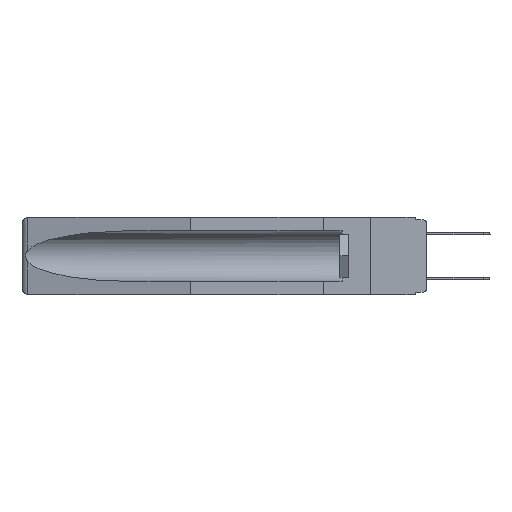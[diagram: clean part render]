
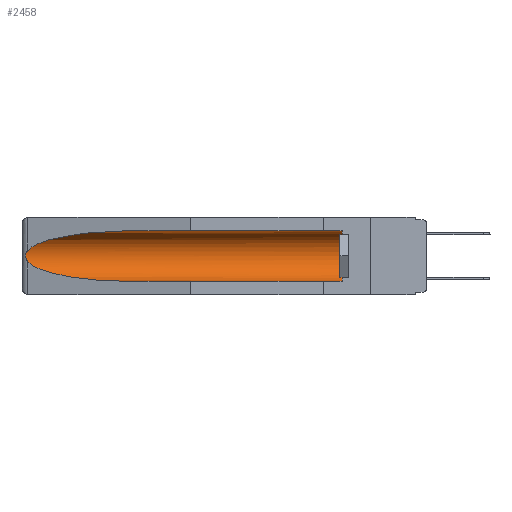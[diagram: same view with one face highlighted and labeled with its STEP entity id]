
A CAD part, left-side view. The second image highlights one B-rep face of the part: STEP entity #2458.
In plain terms, the highlighted cylindrical face has radius 2.857 mm (diameter 5.715 mm), a partial arc.
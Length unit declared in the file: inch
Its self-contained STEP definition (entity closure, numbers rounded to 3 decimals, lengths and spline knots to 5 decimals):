
#445 = CARTESIAN_POINT ( 'NONE',  ( 0.26537, 1.52718, -0.14972 ) ) ;
#566 = CARTESIAN_POINT ( 'NONE',  ( 0.26537, 1.52718, -0.19328 ) ) ;
#662 = VERTEX_POINT ( 'NONE', #4164 ) ;
#961 = EDGE_CURVE ( 'NONE', #3886, #20396, #15527, .T. ) ;
#1002 = CARTESIAN_POINT ( 'NONE',  ( 0.26654, 1.53092, -0.15636 ) ) ;
#1041 = ORIENTED_EDGE ( 'NONE', *, *, #12779, .T. ) ;
#1281 = CARTESIAN_POINT ( 'NONE',  ( 0.155, -0.30754, -0.059 ) ) ;
#2283 = FACE_OUTER_BOUND ( 'NONE', #13771, .T. ) ;
#2370 = ORIENTED_EDGE ( 'NONE', *, *, #7186, .T. ) ;
#2458 = ADVANCED_FACE ( 'NONE', ( #2283 ), #17508, .F. ) ;
#2615 = CARTESIAN_POINT ( 'NONE',  ( 0.155, 1.07973, -0.059 ) ) ;
#2893 = CARTESIAN_POINT ( 'NONE',  ( 0.26597, 1.52961, -0.15275 ) ) ;
#3886 = VERTEX_POINT ( 'NONE', #566 ) ;
#3907 = ORIENTED_EDGE ( 'NONE', *, *, #9377, .F. ) ;
#4164 = CARTESIAN_POINT ( 'NONE',  ( 0.155, 1.07973, -0.059 ) ) ;
#4908 = CARTESIAN_POINT ( 'NONE',  ( 0.26537, 1.52718, -0.14972 ) ) ;
#4993 = CARTESIAN_POINT ( 'NONE',  ( 0.2673, 1.5327, -0.16383 ) ) ;
#7072 = CARTESIAN_POINT ( 'NONE',  ( 0.26655, 1.53094, -0.18657 ) ) ;
#7186 = EDGE_CURVE ( 'NONE', #8641, #662, #25061, .T. ) ;
#7592 = CARTESIAN_POINT ( 'NONE',  ( 0.21114, 1.30732, -0.284 ) ) ;
#8641 = VERTEX_POINT ( 'NONE', #8971 ) ;
#8808 = LINE ( 'NONE', #23559, #21740 ) ;
#8971 = CARTESIAN_POINT ( 'NONE',  ( 0.155, 0.126, -0.059 ) ) ;
#9194 = ORIENTED_EDGE ( 'NONE', *, *, #23063, .T. ) ;
#9377 = EDGE_CURVE ( 'NONE', #14374, #20396, #8808, .T. ) ;
#9402 = CARTESIAN_POINT ( 'NONE',  ( 0.155, -0.30754, -0.1715 ) ) ;
#9589 = CARTESIAN_POINT ( 'NONE',  ( 0.26537, 1.52718, -0.19328 ) ) ;
#9686 = CARTESIAN_POINT ( 'NONE',  ( 0.155, 0.126, -0.284 ) ) ;
#10566 = CARTESIAN_POINT ( 'NONE',  ( 0.155, 1.07973, -0.284 ) ) ;
#11141 = CARTESIAN_POINT ( 'NONE',  ( 0.2673, 1.53269, -0.17917 ) ) ;
#11506 = CARTESIAN_POINT ( 'NONE',  ( 0.26597, 1.5296, -0.19026 ) ) ;
#11543 = VERTEX_POINT ( 'NONE', #21383 ) ;
#12779 = EDGE_CURVE ( 'NONE', #662, #11543, #19136, .T. ) ;
#12822 = CARTESIAN_POINT ( 'NONE',  ( 0.21114, 1.30732, -0.059 ) ) ;
#13771 = EDGE_LOOP ( 'NONE', ( #1041, #25413, #14191, #3907, #9194, #2370 ) ) ;
#14005 = B_SPLINE_CURVE_WITH_KNOTS ( 'NONE', 3,
 ( #4908, #2893, #1002, #4993, #23790, #15584, #11141, #7072, #11506, #19435 ),
 .UNSPECIFIED., .F., .F.,
 ( 4, 2, 2, 2, 4 ),
 ( 0., 0.00029, 0.00058, 0.00087, 0.00117 ),
 .UNSPECIFIED. ) ;
#14191 = ORIENTED_EDGE ( 'NONE', *, *, #961, .T. ) ;
#14374 = VERTEX_POINT ( 'NONE', #9686 ) ;
#15340 = DIRECTION ( 'NONE',  ( 0., 1., 0. ) ) ;
#15527 =( BOUNDED_CURVE ( )  B_SPLINE_CURVE ( 3, ( #9589, #19946, #7592, #18978 ),
 .UNSPECIFIED., .F., .F. ) 
 B_SPLINE_CURVE_WITH_KNOTS ( ( 4, 4 ),
 ( 0.1948, 1.5708 ),
 .UNSPECIFIED. ) 
 CURVE ( )  GEOMETRIC_REPRESENTATION_ITEM ( )  RATIONAL_B_SPLINE_CURVE ( ( 1., 0.848, 0.848, 1. ) ) 
 REPRESENTATION_ITEM ( '' )  );
#15584 = CARTESIAN_POINT ( 'NONE',  ( 0.2675, 1.53308, -0.17534 ) ) ;
#17508 = CYLINDRICAL_SURFACE ( 'NONE', #25681, 0.1125 ) ;
#17677 = VECTOR ( 'NONE', #21809, 39.37008 ) ;
#17998 = DIRECTION ( 'NONE',  ( 0., 1., 0. ) ) ;
#18150 = AXIS2_PLACEMENT_3D ( 'NONE', #26108, #26384, #20142 ) ;
#18978 = CARTESIAN_POINT ( 'NONE',  ( 0.155, 1.07973, -0.284 ) ) ;
#19136 =( BOUNDED_CURVE ( )  B_SPLINE_CURVE ( 3, ( #2615, #12822, #21242, #445 ),
 .UNSPECIFIED., .F., .F. ) 
 B_SPLINE_CURVE_WITH_KNOTS ( ( 4, 4 ),
 ( 4.71239, 6.08839 ),
 .UNSPECIFIED. ) 
 CURVE ( )  GEOMETRIC_REPRESENTATION_ITEM ( )  RATIONAL_B_SPLINE_CURVE ( ( 1., 0.848, 0.848, 1. ) ) 
 REPRESENTATION_ITEM ( '' )  );
#19435 = CARTESIAN_POINT ( 'NONE',  ( 0.26537, 1.52718, -0.19328 ) ) ;
#19946 = CARTESIAN_POINT ( 'NONE',  ( 0.25451, 1.48313, -0.24835 ) ) ;
#19958 = EDGE_CURVE ( 'NONE', #11543, #3886, #14005, .T. ) ;
#20142 = DIRECTION ( 'NONE',  ( 0., 0., 1. ) ) ;
#20396 = VERTEX_POINT ( 'NONE', #10566 ) ;
#21242 = CARTESIAN_POINT ( 'NONE',  ( 0.25451, 1.48313, -0.09465 ) ) ;
#21383 = CARTESIAN_POINT ( 'NONE',  ( 0.26537, 1.52718, -0.14972 ) ) ;
#21740 = VECTOR ( 'NONE', #15340, 39.37008 ) ;
#21809 = DIRECTION ( 'NONE',  ( 0., 1., 0. ) ) ;
#22284 = CIRCLE ( 'NONE', #18150, 0.1125 ) ;
#23017 = DIRECTION ( 'NONE',  ( 0., 0., 1. ) ) ;
#23063 = EDGE_CURVE ( 'NONE', #14374, #8641, #22284, .T. ) ;
#23559 = CARTESIAN_POINT ( 'NONE',  ( 0.155, -0.30754, -0.284 ) ) ;
#23790 = CARTESIAN_POINT ( 'NONE',  ( 0.2675, 1.53308, -0.16763 ) ) ;
#25061 = LINE ( 'NONE', #1281, #17677 ) ;
#25413 = ORIENTED_EDGE ( 'NONE', *, *, #19958, .T. ) ;
#25681 = AXIS2_PLACEMENT_3D ( 'NONE', #9402, #17998, #23017 ) ;
#26108 = CARTESIAN_POINT ( 'NONE',  ( 0.155, 0.126, -0.1715 ) ) ;
#26384 = DIRECTION ( 'NONE',  ( 0., -1., 0. ) ) ;
